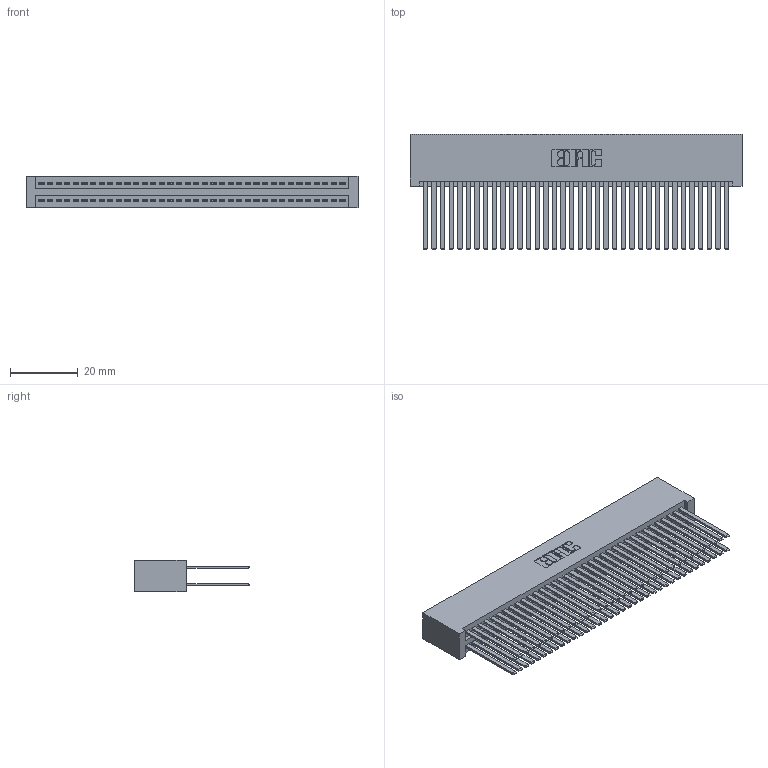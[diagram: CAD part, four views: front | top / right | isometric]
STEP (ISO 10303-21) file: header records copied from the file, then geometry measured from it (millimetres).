
FILE_DESCRIPTION (( 'STEP AP203' ), '1' );
FILE_NAME ('345-072-544-201.STEP', '2018-10-02T07:47:42', ( '' ), ( '' ), 'SwSTEP 2.0', 'SolidWorks 2016', '' );
FILE_SCHEMA (( 'CONFIG_CONTROL_DESIGN' ));
Length unit declared in the file: inch
Products named in the file (3): 345 Part_No Mounting Lugs; 345-292-001_345-293-144; 345-072-544-201
Assembly tree (73 placements, depth 2):
  345-072-544-201
    345 Part_No Mounting Lugs
    345-292-001_345-293-144  x72
Bounding box: 98.04 x 33.96 x 9.4 mm (x, y, z)
Volume: 11093.6 mm3; surface area: 19543.5 mm2
Topology: 73 solids, 73 shells, 3286 faces, 9749 edges, 6402 vertices
Faces by surface type: plane 2164, cylinder 1122
Entity records: 28593 total; most frequent: CARTESIAN_POINT 4796, ORIENTED_EDGE 4730, DIRECTION 4229, EDGE_CURVE 2365, LINE 2101, VECTOR 2101, VERTEX_POINT 1574, AXIS2_PLACEMENT_3D 1064
